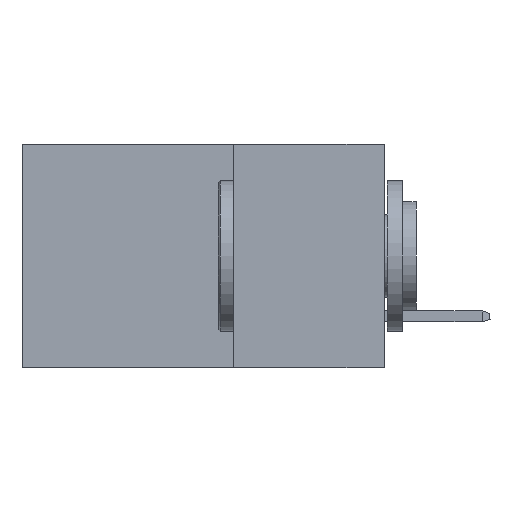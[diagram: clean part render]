
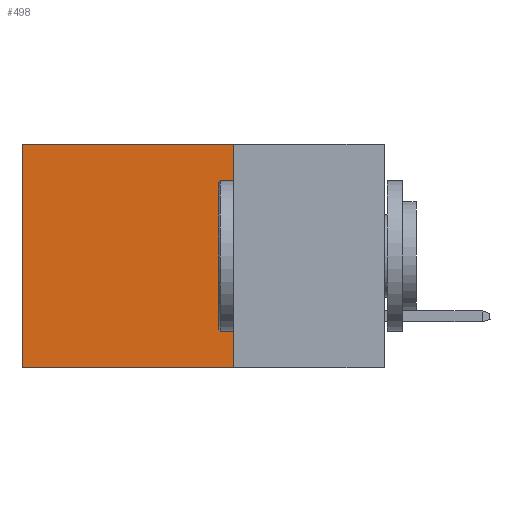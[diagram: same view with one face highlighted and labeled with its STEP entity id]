
A CAD part, left-side view. The second image highlights one B-rep face of the part: STEP entity #498.
In plain terms, the highlighted planar face has unit normal (-1, 0, 0).
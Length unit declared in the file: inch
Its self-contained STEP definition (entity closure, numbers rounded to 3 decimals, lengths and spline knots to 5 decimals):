
#141 = AXIS2_PLACEMENT_3D ( 'NONE', #4733, #6179, #1082 ) ;
#498 = ADVANCED_FACE ( 'NONE', ( #3645 ), #4941, .F. ) ;
#899 = EDGE_CURVE ( 'NONE', #8805, #11035, #12733, .T. ) ;
#1082 = DIRECTION ( 'NONE',  ( 0., 0., -1. ) ) ;
#3007 = DIRECTION ( 'NONE',  ( 0., 0., -1. ) ) ;
#3645 = FACE_OUTER_BOUND ( 'NONE', #15575, .T. ) ;
#3795 = CARTESIAN_POINT ( 'NONE',  ( 0.298, 0.25, -0.37 ) ) ;
#3966 = DIRECTION ( 'NONE',  ( 0., 1., 0. ) ) ;
#4733 = CARTESIAN_POINT ( 'NONE',  ( 0.298, 0.25, 0. ) ) ;
#4787 = VECTOR ( 'NONE', #3007, 39.37008 ) ;
#4941 = PLANE ( 'NONE',  #141 ) ;
#5977 = EDGE_CURVE ( 'NONE', #12922, #8805, #9875, .T. ) ;
#6179 = DIRECTION ( 'NONE',  ( 1., 0., 0. ) ) ;
#6213 = LINE ( 'NONE', #8753, #13966 ) ;
#6536 = ORIENTED_EDGE ( 'NONE', *, *, #15630, .F. ) ;
#8037 = ORIENTED_EDGE ( 'NONE', *, *, #899, .T. ) ;
#8173 = CARTESIAN_POINT ( 'NONE',  ( 0.298, 0.6, -0.37 ) ) ;
#8693 = ORIENTED_EDGE ( 'NONE', *, *, #5977, .T. ) ;
#8753 = CARTESIAN_POINT ( 'NONE',  ( 0.298, 0.25, 0. ) ) ;
#8805 = VERTEX_POINT ( 'NONE', #12972 ) ;
#9875 = LINE ( 'NONE', #14731, #10272 ) ;
#10272 = VECTOR ( 'NONE', #10970, 39.37008 ) ;
#10465 = CARTESIAN_POINT ( 'NONE',  ( 0.298, 0.25, 0. ) ) ;
#10784 = CARTESIAN_POINT ( 'NONE',  ( 0.298, 0.25, -0.37 ) ) ;
#10970 = DIRECTION ( 'NONE',  ( 0., 1., 0. ) ) ;
#11035 = VERTEX_POINT ( 'NONE', #8173 ) ;
#11906 = CARTESIAN_POINT ( 'NONE',  ( 0.298, 0.6, 0. ) ) ;
#12733 = LINE ( 'NONE', #11906, #4787 ) ;
#12922 = VERTEX_POINT ( 'NONE', #10465 ) ;
#12972 = CARTESIAN_POINT ( 'NONE',  ( 0.298, 0.6, 0. ) ) ;
#13058 = VERTEX_POINT ( 'NONE', #10784 ) ;
#13796 = DIRECTION ( 'NONE',  ( 0., 0., -1. ) ) ;
#13907 = EDGE_CURVE ( 'NONE', #12922, #13058, #6213, .T. ) ;
#13966 = VECTOR ( 'NONE', #13796, 39.37008 ) ;
#14150 = LINE ( 'NONE', #3795, #14706 ) ;
#14706 = VECTOR ( 'NONE', #3966, 39.37008 ) ;
#14731 = CARTESIAN_POINT ( 'NONE',  ( 0.298, 0.25, 0. ) ) ;
#14755 = ORIENTED_EDGE ( 'NONE', *, *, #13907, .F. ) ;
#15575 = EDGE_LOOP ( 'NONE', ( #8037, #6536, #14755, #8693 ) ) ;
#15630 = EDGE_CURVE ( 'NONE', #13058, #11035, #14150, .T. ) ;
